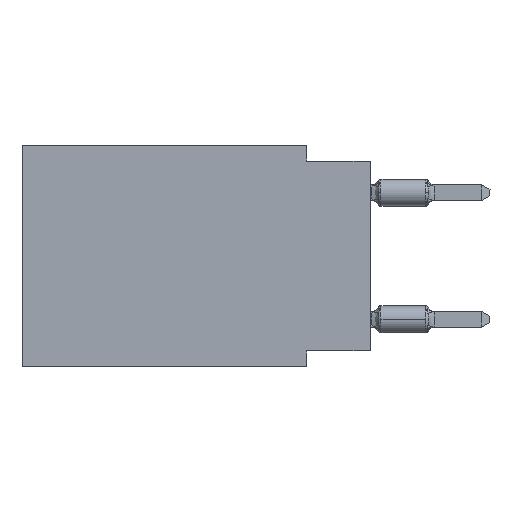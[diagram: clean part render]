
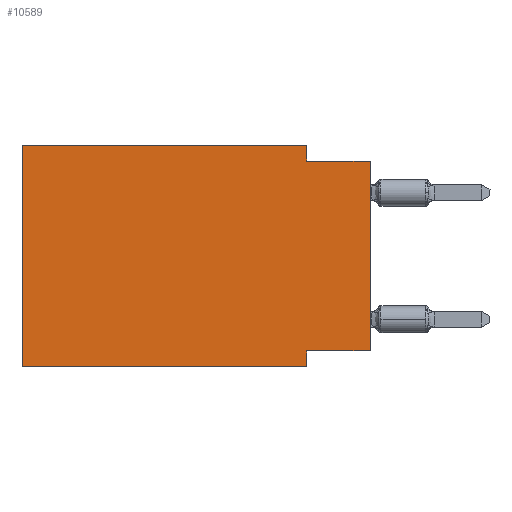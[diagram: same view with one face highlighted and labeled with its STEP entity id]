
A CAD part, left-side view. The second image highlights one B-rep face of the part: STEP entity #10589.
In plain terms, the highlighted planar face has unit normal (-1, 0, 0).
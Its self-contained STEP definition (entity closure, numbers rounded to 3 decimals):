
#2 = ORIENTED_EDGE ( 'NONE', *, *, #13288, .F. ) ;
#34 = VERTEX_POINT ( 'NONE', #10177 ) ;
#1503 = CARTESIAN_POINT ( 'NONE',  ( 0., 2.54, -8.89 ) ) ;
#1941 = VECTOR ( 'NONE', #2825, 1000. ) ;
#2059 = DIRECTION ( 'NONE',  ( 0., -1., 0. ) ) ;
#2404 = CARTESIAN_POINT ( 'NONE',  ( 0., 2.54, -8.255 ) ) ;
#2506 = DIRECTION ( 'NONE',  ( 0., 0., 1. ) ) ;
#2589 = LINE ( 'NONE', #17026, #10143 ) ;
#2614 = EDGE_CURVE ( 'NONE', #9186, #10750, #2589, .T. ) ;
#2724 = CARTESIAN_POINT ( 'NONE',  ( 0., 13.97, 0. ) ) ;
#2825 = DIRECTION ( 'NONE',  ( 0., 0., -1. ) ) ;
#3030 = LINE ( 'NONE', #12099, #10236 ) ;
#4017 = DIRECTION ( 'NONE',  ( 0., 0., -1. ) ) ;
#4032 = VECTOR ( 'NONE', #16266, 1000. ) ;
#4566 = VERTEX_POINT ( 'NONE', #15008 ) ;
#4809 = VECTOR ( 'NONE', #2059, 1000. ) ;
#5419 = CARTESIAN_POINT ( 'NONE',  ( 0., 0., -8.255 ) ) ;
#5486 = FACE_OUTER_BOUND ( 'NONE', #14708, .T. ) ;
#5581 = ORIENTED_EDGE ( 'NONE', *, *, #15718, .T. ) ;
#5845 = VERTEX_POINT ( 'NONE', #13830 ) ;
#6256 = ORIENTED_EDGE ( 'NONE', *, *, #8774, .F. ) ;
#6499 = VECTOR ( 'NONE', #8534, 1000. ) ;
#7230 = VERTEX_POINT ( 'NONE', #10694 ) ;
#7249 = CARTESIAN_POINT ( 'NONE',  ( 0., 13.97, 0. ) ) ;
#7317 = EDGE_CURVE ( 'NONE', #5845, #34, #16312, .T. ) ;
#7830 = DIRECTION ( 'NONE',  ( 1., 0., 0. ) ) ;
#8165 = PLANE ( 'NONE',  #11051 ) ;
#8214 = DIRECTION ( 'NONE',  ( 0., 0., 1. ) ) ;
#8534 = DIRECTION ( 'NONE',  ( 0., -1., 0. ) ) ;
#8774 = EDGE_CURVE ( 'NONE', #15997, #10750, #8972, .T. ) ;
#8972 = LINE ( 'NONE', #16757, #13831 ) ;
#9056 = DIRECTION ( 'NONE',  ( 0., -1., 0. ) ) ;
#9133 = CARTESIAN_POINT ( 'NONE',  ( 0., 2.54, 0. ) ) ;
#9186 = VERTEX_POINT ( 'NONE', #14143 ) ;
#9625 = ORIENTED_EDGE ( 'NONE', *, *, #2614, .T. ) ;
#9942 = VECTOR ( 'NONE', #15701, 1000. ) ;
#10143 = VECTOR ( 'NONE', #2506, 1000. ) ;
#10177 = CARTESIAN_POINT ( 'NONE',  ( 0., 2.54, 0. ) ) ;
#10236 = VECTOR ( 'NONE', #8214, 1000. ) ;
#10589 = ADVANCED_FACE ( 'NONE', ( #5486 ), #8165, .F. ) ;
#10694 = CARTESIAN_POINT ( 'NONE',  ( 0., 13.97, -8.89 ) ) ;
#10750 = VERTEX_POINT ( 'NONE', #15070 ) ;
#10836 = CARTESIAN_POINT ( 'NONE',  ( 0., 2.54, -0.635 ) ) ;
#10912 = LINE ( 'NONE', #1503, #4032 ) ;
#11045 = ORIENTED_EDGE ( 'NONE', *, *, #7317, .F. ) ;
#11051 = AXIS2_PLACEMENT_3D ( 'NONE', #2724, #7830, #4017 ) ;
#11462 = LINE ( 'NONE', #13889, #4809 ) ;
#12099 = CARTESIAN_POINT ( 'NONE',  ( 0., 13.97, 0. ) ) ;
#12883 = EDGE_CURVE ( 'NONE', #15248, #4566, #10912, .T. ) ;
#13288 = EDGE_CURVE ( 'NONE', #7230, #5845, #3030, .T. ) ;
#13355 = ORIENTED_EDGE ( 'NONE', *, *, #14155, .F. ) ;
#13441 = LINE ( 'NONE', #5419, #9942 ) ;
#13672 = ORIENTED_EDGE ( 'NONE', *, *, #14128, .F. ) ;
#13830 = CARTESIAN_POINT ( 'NONE',  ( 0., 13.97, 0. ) ) ;
#13831 = VECTOR ( 'NONE', #9056, 1000. ) ;
#13889 = CARTESIAN_POINT ( 'NONE',  ( 0., 13.97, -8.89 ) ) ;
#14128 = EDGE_CURVE ( 'NONE', #9186, #15248, #13441, .T. ) ;
#14143 = CARTESIAN_POINT ( 'NONE',  ( 0., 0., -8.255 ) ) ;
#14155 = EDGE_CURVE ( 'NONE', #34, #15997, #14741, .T. ) ;
#14245 = ORIENTED_EDGE ( 'NONE', *, *, #12883, .F. ) ;
#14708 = EDGE_LOOP ( 'NONE', ( #9625, #6256, #13355, #11045, #2, #5581, #14245, #13672 ) ) ;
#14741 = LINE ( 'NONE', #9133, #1941 ) ;
#15008 = CARTESIAN_POINT ( 'NONE',  ( 0., 2.54, -8.89 ) ) ;
#15070 = CARTESIAN_POINT ( 'NONE',  ( 0., 0., -0.635 ) ) ;
#15248 = VERTEX_POINT ( 'NONE', #2404 ) ;
#15701 = DIRECTION ( 'NONE',  ( 0., 1., 0. ) ) ;
#15718 = EDGE_CURVE ( 'NONE', #7230, #4566, #11462, .T. ) ;
#15997 = VERTEX_POINT ( 'NONE', #10836 ) ;
#16266 = DIRECTION ( 'NONE',  ( 0., 0., -1. ) ) ;
#16312 = LINE ( 'NONE', #7249, #6499 ) ;
#16757 = CARTESIAN_POINT ( 'NONE',  ( 0., 0., -0.635 ) ) ;
#17026 = CARTESIAN_POINT ( 'NONE',  ( 0., 0., 0. ) ) ;
